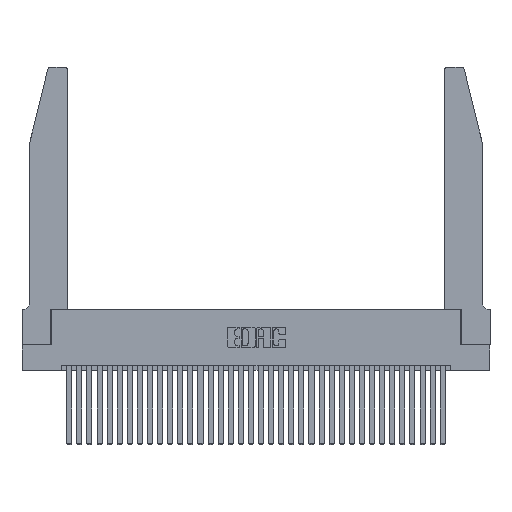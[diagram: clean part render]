
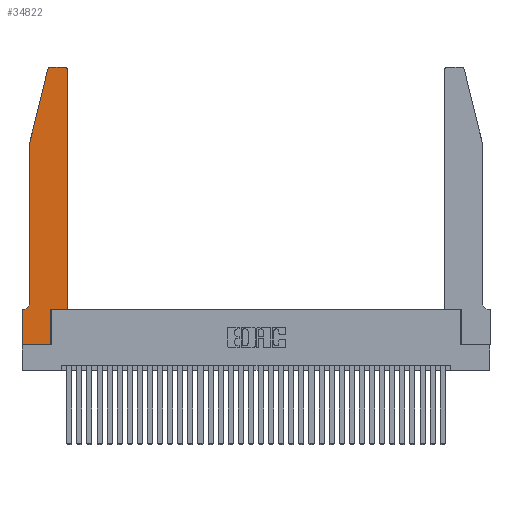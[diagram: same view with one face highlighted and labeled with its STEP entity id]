
A CAD part, top view. The second image highlights one B-rep face of the part: STEP entity #34822.
In plain terms, the highlighted planar face has unit normal (0, 0, 1).
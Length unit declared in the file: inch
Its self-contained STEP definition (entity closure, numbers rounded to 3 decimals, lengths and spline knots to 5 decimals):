
#268 = CARTESIAN_POINT ( 'NONE',  ( 0., 0.35, 0.37 ) ) ;
#365 = LINE ( 'NONE', #31014, #13930 ) ;
#559 = ORIENTED_EDGE ( 'NONE', *, *, #3634, .T. ) ;
#636 = DIRECTION ( 'NONE',  ( 0., 0., -1. ) ) ;
#945 = VERTEX_POINT ( 'NONE', #8784 ) ;
#1010 = CARTESIAN_POINT ( 'NONE',  ( 0.4205, 2.75, 0.37 ) ) ;
#1145 = DIRECTION ( 'NONE',  ( 0., -1., 0. ) ) ;
#1264 = CARTESIAN_POINT ( 'NONE',  ( 0., 0., 0.37 ) ) ;
#1431 = ORIENTED_EDGE ( 'NONE', *, *, #32040, .T. ) ;
#2623 = ORIENTED_EDGE ( 'NONE', *, *, #23042, .T. ) ;
#2771 = EDGE_CURVE ( 'NONE', #945, #4738, #16728, .T. ) ;
#2894 = VECTOR ( 'NONE', #33004, 39.37008 ) ;
#2985 = ORIENTED_EDGE ( 'NONE', *, *, #30812, .T. ) ;
#3061 = ORIENTED_EDGE ( 'NONE', *, *, #19212, .T. ) ;
#3274 = DIRECTION ( 'NONE',  ( 1., 0., 0. ) ) ;
#3311 = DIRECTION ( 'NONE',  ( -1., 0., 0. ) ) ;
#3342 = DIRECTION ( 'NONE',  ( 1., 0., 0. ) ) ;
#3567 = VERTEX_POINT ( 'NONE', #1264 ) ;
#3634 = EDGE_CURVE ( 'NONE', #33399, #21913, #11571, .T. ) ;
#4083 = ORIENTED_EDGE ( 'NONE', *, *, #19994, .T. ) ;
#4132 = CARTESIAN_POINT ( 'NONE',  ( 0.4505, 0.35, 0.37 ) ) ;
#4738 = VERTEX_POINT ( 'NONE', #18886 ) ;
#6290 = VECTOR ( 'NONE', #19490, 39.37008 ) ;
#6676 = CARTESIAN_POINT ( 'NONE',  ( 0.0755, 2., 0.37 ) ) ;
#7848 = ORIENTED_EDGE ( 'NONE', *, *, #14132, .T. ) ;
#7932 = CARTESIAN_POINT ( 'NONE',  ( 0., 0., 0.37 ) ) ;
#8559 = VECTOR ( 'NONE', #25111, 39.37008 ) ;
#8784 = CARTESIAN_POINT ( 'NONE',  ( 0.0755, 0.42, 0.37 ) ) ;
#9145 = LINE ( 'NONE', #7932, #16797 ) ;
#9363 = CARTESIAN_POINT ( 'NONE',  ( 0.4505, 2.72, 0.37 ) ) ;
#9414 = LINE ( 'NONE', #22438, #8559 ) ;
#11571 = CIRCLE ( 'NONE', #17607, 0.03 ) ;
#12307 = CARTESIAN_POINT ( 'NONE',  ( 0.0755, 2., 0.37 ) ) ;
#12638 = AXIS2_PLACEMENT_3D ( 'NONE', #13787, #636, #3311 ) ;
#13662 = PLANE ( 'NONE',  #34260 ) ;
#13787 = CARTESIAN_POINT ( 'NONE',  ( 0.0055, 0.42, 0.37 ) ) ;
#13930 = VECTOR ( 'NONE', #1145, 39.37008 ) ;
#13934 = EDGE_LOOP ( 'NONE', ( #2985, #30988, #21251, #2623, #17292, #1431, #3061, #32168, #14553, #4083, #7848, #559 ) ) ;
#13983 = DIRECTION ( 'NONE',  ( 0., 0., 1. ) ) ;
#14132 = EDGE_CURVE ( 'NONE', #32090, #33399, #22790, .T. ) ;
#14135 = VERTEX_POINT ( 'NONE', #33971 ) ;
#14162 = DIRECTION ( 'NONE',  ( 0., -1., 0. ) ) ;
#14203 = CARTESIAN_POINT ( 'NONE',  ( 0.284, 2.75, 0.37 ) ) ;
#14553 = ORIENTED_EDGE ( 'NONE', *, *, #34350, .T. ) ;
#14678 = VERTEX_POINT ( 'NONE', #31493 ) ;
#14789 = DIRECTION ( 'NONE',  ( 0., 0., 1. ) ) ;
#14846 = LINE ( 'NONE', #19611, #6290 ) ;
#15207 = LINE ( 'NONE', #21743, #34146 ) ;
#15767 = LINE ( 'NONE', #20205, #27474 ) ;
#15981 = VECTOR ( 'NONE', #31157, 39.37008 ) ;
#16287 = EDGE_CURVE ( 'NONE', #3567, #14678, #9145, .T. ) ;
#16543 = EDGE_CURVE ( 'NONE', #14135, #23087, #24761, .T. ) ;
#16728 = CIRCLE ( 'NONE', #12638, 0.07 ) ;
#16797 = VECTOR ( 'NONE', #3342, 39.37008 ) ;
#17292 = ORIENTED_EDGE ( 'NONE', *, *, #2771, .T. ) ;
#17467 = DIRECTION ( 'NONE',  ( 1., 0., 0. ) ) ;
#17607 = AXIS2_PLACEMENT_3D ( 'NONE', #20027, #14789, #17467 ) ;
#18886 = CARTESIAN_POINT ( 'NONE',  ( 0.0055, 0.35, 0.37 ) ) ;
#19167 = DIRECTION ( 'NONE',  ( 0., 0., 1. ) ) ;
#19212 = EDGE_CURVE ( 'NONE', #34600, #3567, #31369, .T. ) ;
#19490 = DIRECTION ( 'NONE',  ( -1., 0., 0. ) ) ;
#19611 = CARTESIAN_POINT ( 'NONE',  ( 0.0755, 0.35, 0.37 ) ) ;
#19656 = CARTESIAN_POINT ( 'NONE',  ( 0., 0., 0.37 ) ) ;
#19994 = EDGE_CURVE ( 'NONE', #33849, #32090, #9414, .T. ) ;
#20027 = CARTESIAN_POINT ( 'NONE',  ( 0.4205, 2.72, 0.37 ) ) ;
#20205 = CARTESIAN_POINT ( 'NONE',  ( 0.2605, 2.75, 0.37 ) ) ;
#20667 = AXIS2_PLACEMENT_3D ( 'NONE', #27491, #13983, #3274 ) ;
#21251 = ORIENTED_EDGE ( 'NONE', *, *, #16543, .T. ) ;
#21743 = CARTESIAN_POINT ( 'NONE',  ( 0.2865, 0.35, 0.37 ) ) ;
#21913 = VERTEX_POINT ( 'NONE', #1010 ) ;
#22162 = VERTEX_POINT ( 'NONE', #14203 ) ;
#22438 = CARTESIAN_POINT ( 'NONE',  ( 0.4505, 0.35, 0.37 ) ) ;
#22790 = LINE ( 'NONE', #27562, #2894 ) ;
#23042 = EDGE_CURVE ( 'NONE', #23087, #945, #365, .T. ) ;
#23087 = VERTEX_POINT ( 'NONE', #6676 ) ;
#24159 = VECTOR ( 'NONE', #14162, 39.37008 ) ;
#24642 = DIRECTION ( 'NONE',  ( 0., 1., 0. ) ) ;
#24761 = LINE ( 'NONE', #12307, #15981 ) ;
#24796 = DIRECTION ( 'NONE',  ( 1., 0., 0. ) ) ;
#25111 = DIRECTION ( 'NONE',  ( 1., 0., 0. ) ) ;
#27474 = VECTOR ( 'NONE', #33409, 39.37008 ) ;
#27491 = CARTESIAN_POINT ( 'NONE',  ( 0.284, 2.72, 0.37 ) ) ;
#27562 = CARTESIAN_POINT ( 'NONE',  ( 0.4505, 0.35, 0.37 ) ) ;
#28682 = CIRCLE ( 'NONE', #20667, 0.03 ) ;
#29541 = CARTESIAN_POINT ( 'NONE',  ( 0.2865, 0.35, 0.37 ) ) ;
#30812 = EDGE_CURVE ( 'NONE', #21913, #22162, #15767, .T. ) ;
#30988 = ORIENTED_EDGE ( 'NONE', *, *, #34001, .T. ) ;
#31014 = CARTESIAN_POINT ( 'NONE',  ( 0.0755, 2., 0.37 ) ) ;
#31157 = DIRECTION ( 'NONE',  ( -0.239, -0.971, 0. ) ) ;
#31369 = LINE ( 'NONE', #19656, #24159 ) ;
#31493 = CARTESIAN_POINT ( 'NONE',  ( 0.2865, 0., 0.37 ) ) ;
#32040 = EDGE_CURVE ( 'NONE', #4738, #34600, #14846, .T. ) ;
#32090 = VERTEX_POINT ( 'NONE', #4132 ) ;
#32168 = ORIENTED_EDGE ( 'NONE', *, *, #16287, .T. ) ;
#32413 = FACE_OUTER_BOUND ( 'NONE', #13934, .T. ) ;
#33004 = DIRECTION ( 'NONE',  ( 0., 1., 0. ) ) ;
#33399 = VERTEX_POINT ( 'NONE', #9363 ) ;
#33409 = DIRECTION ( 'NONE',  ( -1., 0., 0. ) ) ;
#33849 = VERTEX_POINT ( 'NONE', #29541 ) ;
#33971 = CARTESIAN_POINT ( 'NONE',  ( 0.25487, 2.72718, 0.37 ) ) ;
#34001 = EDGE_CURVE ( 'NONE', #22162, #14135, #28682, .T. ) ;
#34146 = VECTOR ( 'NONE', #24642, 39.37008 ) ;
#34260 = AXIS2_PLACEMENT_3D ( 'NONE', #268, #19167, #24796 ) ;
#34350 = EDGE_CURVE ( 'NONE', #14678, #33849, #15207, .T. ) ;
#34600 = VERTEX_POINT ( 'NONE', #34885 ) ;
#34822 = ADVANCED_FACE ( 'NONE', ( #32413 ), #13662, .T. ) ;
#34885 = CARTESIAN_POINT ( 'NONE',  ( 0., 0.35, 0.37 ) ) ;
